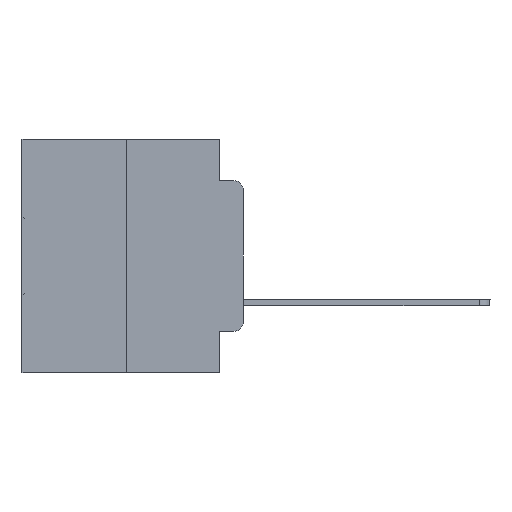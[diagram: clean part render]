
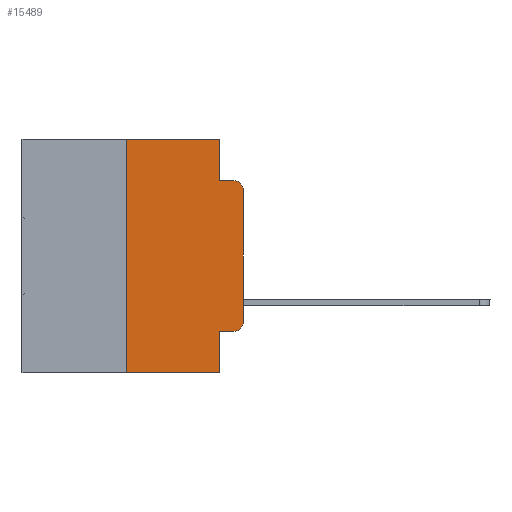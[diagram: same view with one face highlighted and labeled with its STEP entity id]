
A CAD part, left-side view. The second image highlights one B-rep face of the part: STEP entity #15489.
In plain terms, the highlighted planar face has unit normal (-1, 0, 0).
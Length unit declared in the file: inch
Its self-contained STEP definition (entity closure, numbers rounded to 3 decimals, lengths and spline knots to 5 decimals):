
#116 = ORIENTED_EDGE ( 'NONE', *, *, #7887, .F. ) ;
#481 = DIRECTION ( 'NONE',  ( 0., -1., 0. ) ) ;
#804 = DIRECTION ( 'NONE',  ( 1., 0., 0. ) ) ;
#840 = EDGE_LOOP ( 'NONE', ( #26158, #16975, #116, #31351, #10781, #7203, #5353, #31301, #6600, #16420 ) ) ;
#980 = CARTESIAN_POINT ( 'NONE',  ( 0., 0.473, 0. ) ) ;
#1684 = DIRECTION ( 'NONE',  ( 0., 0., 1. ) ) ;
#2294 = EDGE_CURVE ( 'NONE', #17675, #21738, #13509, .T. ) ;
#2485 = DIRECTION ( 'NONE',  ( 0., -1., 0. ) ) ;
#2637 = EDGE_CURVE ( 'NONE', #25871, #17675, #29437, .T. ) ;
#3578 = VERTEX_POINT ( 'NONE', #15263 ) ;
#3654 = VECTOR ( 'NONE', #1684, 39.37008 ) ;
#3804 = CARTESIAN_POINT ( 'NONE',  ( 0., 0.051, -0.0885 ) ) ;
#3971 = VECTOR ( 'NONE', #14536, 39.37008 ) ;
#4011 = VECTOR ( 'NONE', #23274, 39.37008 ) ;
#4567 = LINE ( 'NONE', #26734, #21363 ) ;
#5353 = ORIENTED_EDGE ( 'NONE', *, *, #6788, .T. ) ;
#6310 = CARTESIAN_POINT ( 'NONE',  ( 0., 0.02, -0.1085 ) ) ;
#6354 = CARTESIAN_POINT ( 'NONE',  ( 0., 0.051, -0.4115 ) ) ;
#6600 = ORIENTED_EDGE ( 'NONE', *, *, #26836, .T. ) ;
#6788 = EDGE_CURVE ( 'NONE', #29608, #29262, #4567, .T. ) ;
#6881 = CARTESIAN_POINT ( 'NONE',  ( 0., 0.051, 0. ) ) ;
#7165 = DIRECTION ( 'NONE',  ( 0., 0., -1. ) ) ;
#7203 = ORIENTED_EDGE ( 'NONE', *, *, #22775, .F. ) ;
#7502 = CARTESIAN_POINT ( 'NONE',  ( 0., 0.051, 0. ) ) ;
#7584 = EDGE_CURVE ( 'NONE', #10281, #31200, #9618, .T. ) ;
#7597 = CARTESIAN_POINT ( 'NONE',  ( 0., 0.02, -0.0885 ) ) ;
#7887 = EDGE_CURVE ( 'NONE', #31200, #21738, #25672, .T. ) ;
#8642 = DIRECTION ( 'NONE',  ( 0., 0., -1. ) ) ;
#9464 = VECTOR ( 'NONE', #23436, 39.37008 ) ;
#9618 = LINE ( 'NONE', #6881, #3971 ) ;
#10281 = VERTEX_POINT ( 'NONE', #7502 ) ;
#10781 = ORIENTED_EDGE ( 'NONE', *, *, #27591, .F. ) ;
#11495 = AXIS2_PLACEMENT_3D ( 'NONE', #6310, #25756, #16028 ) ;
#12010 = EDGE_CURVE ( 'NONE', #3578, #25871, #13259, .T. ) ;
#12029 = DIRECTION ( 'NONE',  ( -1., 0., 0. ) ) ;
#12348 = CARTESIAN_POINT ( 'NONE',  ( 0., 0.02, -0.3915 ) ) ;
#12523 = DIRECTION ( 'NONE',  ( 0., 0., 1. ) ) ;
#13259 = CIRCLE ( 'NONE', #28535, 0.02 ) ;
#13509 = CIRCLE ( 'NONE', #11495, 0.02 ) ;
#14475 = CARTESIAN_POINT ( 'NONE',  ( 0., 0.25, -0.5 ) ) ;
#14536 = DIRECTION ( 'NONE',  ( 0., 0., -1. ) ) ;
#14699 = CARTESIAN_POINT ( 'NONE',  ( 0., 0.473, 0. ) ) ;
#15186 = FACE_OUTER_BOUND ( 'NONE', #840, .T. ) ;
#15263 = CARTESIAN_POINT ( 'NONE',  ( 0., 0.02, -0.4115 ) ) ;
#15489 = ADVANCED_FACE ( 'NONE', ( #15186 ), #29104, .F. ) ;
#15579 = CARTESIAN_POINT ( 'NONE',  ( 0., 0., -0.1085 ) ) ;
#16028 = DIRECTION ( 'NONE',  ( 0., 0., -1. ) ) ;
#16075 = LINE ( 'NONE', #6354, #9464 ) ;
#16420 = ORIENTED_EDGE ( 'NONE', *, *, #12010, .T. ) ;
#16975 = ORIENTED_EDGE ( 'NONE', *, *, #2294, .T. ) ;
#17098 = VERTEX_POINT ( 'NONE', #22513 ) ;
#17675 = VERTEX_POINT ( 'NONE', #15579 ) ;
#18450 = CARTESIAN_POINT ( 'NONE',  ( 0., 0.25, 0. ) ) ;
#19138 = AXIS2_PLACEMENT_3D ( 'NONE', #980, #804, #8642 ) ;
#19676 = CARTESIAN_POINT ( 'NONE',  ( 0., 0., 0. ) ) ;
#21034 = CARTESIAN_POINT ( 'NONE',  ( 0., 0.051, -0.0885 ) ) ;
#21158 = LINE ( 'NONE', #18450, #3654 ) ;
#21179 = EDGE_CURVE ( 'NONE', #23394, #29262, #26617, .T. ) ;
#21363 = VECTOR ( 'NONE', #2485, 39.37008 ) ;
#21672 = CARTESIAN_POINT ( 'NONE',  ( 0., 0.051, 0. ) ) ;
#21738 = VERTEX_POINT ( 'NONE', #7597 ) ;
#21919 = DIRECTION ( 'NONE',  ( 0., 0., -1. ) ) ;
#22513 = CARTESIAN_POINT ( 'NONE',  ( 0., 0.25, 0. ) ) ;
#22528 = LINE ( 'NONE', #14699, #24264 ) ;
#22775 = EDGE_CURVE ( 'NONE', #29608, #17098, #21158, .T. ) ;
#23274 = DIRECTION ( 'NONE',  ( 0., -1., 0. ) ) ;
#23394 = VERTEX_POINT ( 'NONE', #23499 ) ;
#23436 = DIRECTION ( 'NONE',  ( 0., -1., 0. ) ) ;
#23499 = CARTESIAN_POINT ( 'NONE',  ( 0., 0.051, -0.4115 ) ) ;
#24264 = VECTOR ( 'NONE', #481, 39.37008 ) ;
#24960 = VECTOR ( 'NONE', #7165, 39.37008 ) ;
#25672 = LINE ( 'NONE', #3804, #4011 ) ;
#25756 = DIRECTION ( 'NONE',  ( -1., 0., 0. ) ) ;
#25871 = VERTEX_POINT ( 'NONE', #27097 ) ;
#26158 = ORIENTED_EDGE ( 'NONE', *, *, #2637, .T. ) ;
#26430 = VECTOR ( 'NONE', #12523, 39.37008 ) ;
#26617 = LINE ( 'NONE', #21672, #24960 ) ;
#26734 = CARTESIAN_POINT ( 'NONE',  ( 0., 0.473, -0.5 ) ) ;
#26836 = EDGE_CURVE ( 'NONE', #23394, #3578, #16075, .T. ) ;
#26999 = CARTESIAN_POINT ( 'NONE',  ( 0., 0.051, -0.5 ) ) ;
#27097 = CARTESIAN_POINT ( 'NONE',  ( 0., 0., -0.3915 ) ) ;
#27591 = EDGE_CURVE ( 'NONE', #17098, #10281, #22528, .T. ) ;
#28535 = AXIS2_PLACEMENT_3D ( 'NONE', #12348, #12029, #21919 ) ;
#29104 = PLANE ( 'NONE',  #19138 ) ;
#29262 = VERTEX_POINT ( 'NONE', #26999 ) ;
#29437 = LINE ( 'NONE', #19676, #26430 ) ;
#29608 = VERTEX_POINT ( 'NONE', #14475 ) ;
#31200 = VERTEX_POINT ( 'NONE', #21034 ) ;
#31301 = ORIENTED_EDGE ( 'NONE', *, *, #21179, .F. ) ;
#31351 = ORIENTED_EDGE ( 'NONE', *, *, #7584, .F. ) ;
